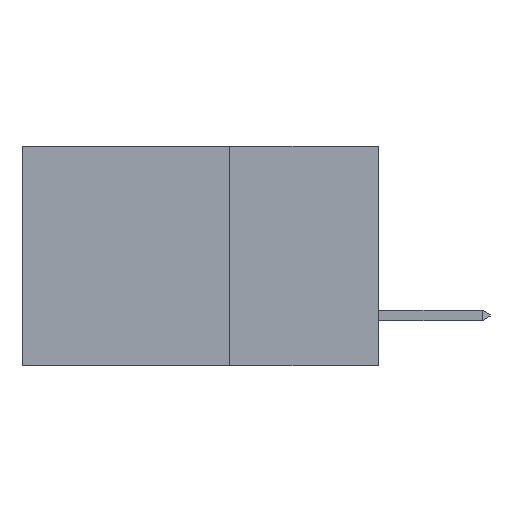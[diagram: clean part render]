
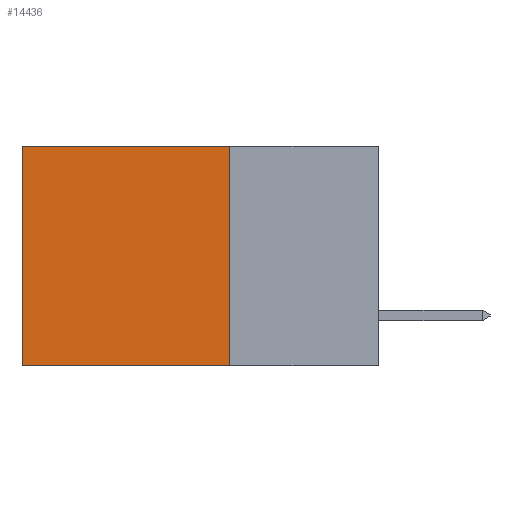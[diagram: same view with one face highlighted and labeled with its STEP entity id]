
A CAD part, left-side view. The second image highlights one B-rep face of the part: STEP entity #14436.
In plain terms, the highlighted planar face has unit normal (-1, 0, 0).
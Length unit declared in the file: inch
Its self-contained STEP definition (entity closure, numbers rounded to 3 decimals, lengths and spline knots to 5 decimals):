
#39 = EDGE_LOOP ( 'NONE', ( #3685, #18971, #4119, #283 ) ) ;
#165 = DIRECTION ( 'NONE',  ( 0., 1., 0. ) ) ;
#283 = ORIENTED_EDGE ( 'NONE', *, *, #4983, .T. ) ;
#1285 = DIRECTION ( 'NONE',  ( 0., 0., -1. ) ) ;
#1529 = LINE ( 'NONE', #19632, #12837 ) ;
#1623 = CARTESIAN_POINT ( 'NONE',  ( 0.298, 0.25, 0. ) ) ;
#3685 = ORIENTED_EDGE ( 'NONE', *, *, #17258, .T. ) ;
#3910 = DIRECTION ( 'NONE',  ( 0., 1., 0. ) ) ;
#4119 = ORIENTED_EDGE ( 'NONE', *, *, #18882, .F. ) ;
#4713 = VERTEX_POINT ( 'NONE', #11143 ) ;
#4895 = VECTOR ( 'NONE', #165, 39.37008 ) ;
#4983 = EDGE_CURVE ( 'NONE', #9454, #4713, #12983, .T. ) ;
#5852 = AXIS2_PLACEMENT_3D ( 'NONE', #5915, #8978, #19415 ) ;
#5915 = CARTESIAN_POINT ( 'NONE',  ( 0.298, 0.25, 0. ) ) ;
#6404 = CARTESIAN_POINT ( 'NONE',  ( 0.298, 0.25, -0.37 ) ) ;
#7879 = CARTESIAN_POINT ( 'NONE',  ( 0.298, 0.25, -0.37 ) ) ;
#8719 = LINE ( 'NONE', #12062, #12288 ) ;
#8978 = DIRECTION ( 'NONE',  ( 1., 0., 0. ) ) ;
#9191 = DIRECTION ( 'NONE',  ( 0., 0., -1. ) ) ;
#9454 = VERTEX_POINT ( 'NONE', #12008 ) ;
#10409 = PLANE ( 'NONE',  #5852 ) ;
#10771 = CARTESIAN_POINT ( 'NONE',  ( 0.298, 0.6, -0.37 ) ) ;
#11143 = CARTESIAN_POINT ( 'NONE',  ( 0.298, 0.6, 0. ) ) ;
#11594 = VERTEX_POINT ( 'NONE', #6404 ) ;
#12008 = CARTESIAN_POINT ( 'NONE',  ( 0.298, 0.25, 0. ) ) ;
#12062 = CARTESIAN_POINT ( 'NONE',  ( 0.298, 0.25, 0. ) ) ;
#12288 = VECTOR ( 'NONE', #1285, 39.37008 ) ;
#12837 = VECTOR ( 'NONE', #9191, 39.37008 ) ;
#12983 = LINE ( 'NONE', #1623, #16509 ) ;
#13885 = VERTEX_POINT ( 'NONE', #10771 ) ;
#14436 = ADVANCED_FACE ( 'NONE', ( #15793 ), #10409, .F. ) ;
#15793 = FACE_OUTER_BOUND ( 'NONE', #39, .T. ) ;
#16509 = VECTOR ( 'NONE', #3910, 39.37008 ) ;
#16974 = LINE ( 'NONE', #7879, #4895 ) ;
#17258 = EDGE_CURVE ( 'NONE', #4713, #13885, #1529, .T. ) ;
#18882 = EDGE_CURVE ( 'NONE', #9454, #11594, #8719, .T. ) ;
#18971 = ORIENTED_EDGE ( 'NONE', *, *, #19045, .F. ) ;
#19045 = EDGE_CURVE ( 'NONE', #11594, #13885, #16974, .T. ) ;
#19415 = DIRECTION ( 'NONE',  ( 0., 0., -1. ) ) ;
#19632 = CARTESIAN_POINT ( 'NONE',  ( 0.298, 0.6, 0. ) ) ;
